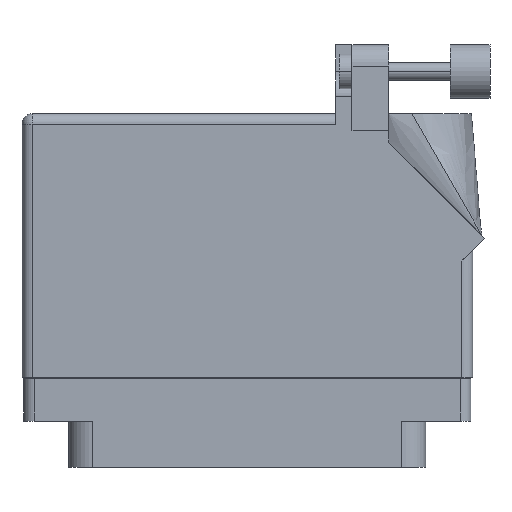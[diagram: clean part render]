
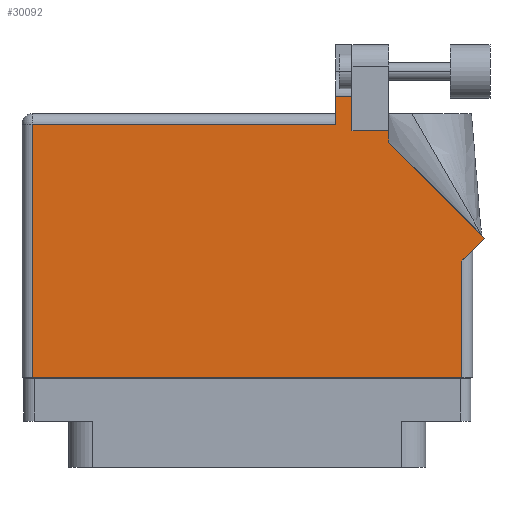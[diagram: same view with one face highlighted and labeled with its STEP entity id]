
A CAD part, front view. The second image highlights one B-rep face of the part: STEP entity #30092.
In plain terms, the highlighted face is planar.
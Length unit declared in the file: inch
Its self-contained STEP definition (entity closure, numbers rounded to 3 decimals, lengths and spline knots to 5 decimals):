
#143 = DIRECTION ( 'NONE',  ( -1., 0., 0. ) ) ;
#302 = EDGE_CURVE ( 'NONE', #26790, #39023, #39555, .T. ) ;
#1346 = EDGE_CURVE ( 'NONE', #25140, #21363, #42938, .T. ) ;
#1649 = EDGE_CURVE ( 'NONE', #23870, #14553, #26015, .T. ) ;
#1766 = ORIENTED_EDGE ( 'NONE', *, *, #33555, .T. ) ;
#2999 = ORIENTED_EDGE ( 'NONE', *, *, #47303, .T. ) ;
#3070 = DIRECTION ( 'NONE',  ( -1., 0., 0. ) ) ;
#3093 = EDGE_LOOP ( 'NONE', ( #38251, #18678, #31161, #1766, #7810, #27589, #23297, #26671, #46212, #2999, #3477 ) ) ;
#3477 = ORIENTED_EDGE ( 'NONE', *, *, #1346, .T. ) ;
#3501 = EDGE_CURVE ( 'NONE', #41612, #23870, #7761, .T. ) ;
#4159 = LINE ( 'NONE', #20643, #32594 ) ;
#5684 = LINE ( 'NONE', #46859, #42906 ) ;
#7761 = LINE ( 'NONE', #21615, #10096 ) ;
#7810 = ORIENTED_EDGE ( 'NONE', *, *, #3501, .T. ) ;
#8825 = CARTESIAN_POINT ( 'NONE',  ( 0.513, 1.5315, 0.455 ) ) ;
#8990 = CARTESIAN_POINT ( 'NONE',  ( 0.82, 1.33, 0.455 ) ) ;
#9104 = CARTESIAN_POINT ( 'NONE',  ( -1.306, -0.1, 0.455 ) ) ;
#10096 = VECTOR ( 'NONE', #36224, 39.37008 ) ;
#10325 = CARTESIAN_POINT ( 'NONE',  ( -1.306, 1.43, 0.455 ) ) ;
#10364 = LINE ( 'NONE', #22560, #47624 ) ;
#11052 = CARTESIAN_POINT ( 'NONE',  ( 0.513, 1.43, 0.455 ) ) ;
#11156 = CARTESIAN_POINT ( 'NONE',  ( 0.82, 1.33, 0.455 ) ) ;
#11971 = CARTESIAN_POINT ( 'NONE',  ( 0.607, 1.5315, 0.455 ) ) ;
#13573 = DIRECTION ( 'NONE',  ( 1., 0., 0. ) ) ;
#14553 = VERTEX_POINT ( 'NONE', #41869 ) ;
#15030 = DIRECTION ( 'NONE',  ( 0., -1., 0. ) ) ;
#15648 = VECTOR ( 'NONE', #45522, 39.37008 ) ;
#17263 = DIRECTION ( 'NONE',  ( -0.707, 0.707, 0. ) ) ;
#17900 = CARTESIAN_POINT ( 'NONE',  ( 1.37671, 0.70771, 0.455 ) ) ;
#18544 = DIRECTION ( 'NONE',  ( 0., 1., 0. ) ) ;
#18678 = ORIENTED_EDGE ( 'NONE', *, *, #45038, .T. ) ;
#19804 = VERTEX_POINT ( 'NONE', #17900 ) ;
#20394 = EDGE_CURVE ( 'NONE', #19804, #39127, #5684, .T. ) ;
#20643 = CARTESIAN_POINT ( 'NONE',  ( 0.93777, 1.5315, 0.455 ) ) ;
#20734 = CARTESIAN_POINT ( 'NONE',  ( 0.513, 1.368, 0.455 ) ) ;
#21363 = VERTEX_POINT ( 'NONE', #35754 ) ;
#21615 = CARTESIAN_POINT ( 'NONE',  ( -1.244, -0.1, 0.455 ) ) ;
#22560 = CARTESIAN_POINT ( 'NONE',  ( 0.607, 1.33, 0.455 ) ) ;
#23103 = VECTOR ( 'NONE', #13573, 39.37008 ) ;
#23297 = ORIENTED_EDGE ( 'NONE', *, *, #46153, .T. ) ;
#23406 = DIRECTION ( 'NONE',  ( -1., 0., 0. ) ) ;
#23870 = VERTEX_POINT ( 'NONE', #38397 ) ;
#24370 = VECTOR ( 'NONE', #15030, 39.37008 ) ;
#24628 = LINE ( 'NONE', #30578, #34501 ) ;
#25140 = VERTEX_POINT ( 'NONE', #8990 ) ;
#26015 = LINE ( 'NONE', #9104, #23103 ) ;
#26671 = ORIENTED_EDGE ( 'NONE', *, *, #31814, .T. ) ;
#26790 = VERTEX_POINT ( 'NONE', #8825 ) ;
#27062 = VECTOR ( 'NONE', #30600, 39.37008 ) ;
#27589 = ORIENTED_EDGE ( 'NONE', *, *, #1649, .T. ) ;
#27820 = CARTESIAN_POINT ( 'NONE',  ( 0.82, 1.26442, 0.455 ) ) ;
#27990 = DIRECTION ( 'NONE',  ( 0., 1., 0. ) ) ;
#29434 = VECTOR ( 'NONE', #27990, 39.37008 ) ;
#29480 = LINE ( 'NONE', #37997, #15648 ) ;
#30092 = ADVANCED_FACE ( 'NONE', ( #32371 ), #36321, .F. ) ;
#30578 = CARTESIAN_POINT ( 'NONE',  ( -1.306, 1.368, 0.455 ) ) ;
#30600 = DIRECTION ( 'NONE',  ( 0., 1., 0. ) ) ;
#31161 = ORIENTED_EDGE ( 'NONE', *, *, #302, .T. ) ;
#31619 = EDGE_CURVE ( 'NONE', #21363, #41381, #10364, .T. ) ;
#31814 = EDGE_CURVE ( 'NONE', #38472, #19804, #29480, .T. ) ;
#32371 = FACE_OUTER_BOUND ( 'NONE', #3093, .T. ) ;
#32594 = VECTOR ( 'NONE', #43076, 39.37008 ) ;
#32926 = LINE ( 'NONE', #34649, #27062 ) ;
#33509 = LINE ( 'NONE', #27820, #29434 ) ;
#33555 = EDGE_CURVE ( 'NONE', #39023, #41612, #24628, .T. ) ;
#34501 = VECTOR ( 'NONE', #23406, 39.37008 ) ;
#34649 = CARTESIAN_POINT ( 'NONE',  ( 1.244, 0.637, 0.455 ) ) ;
#35754 = CARTESIAN_POINT ( 'NONE',  ( 0.607, 1.33, 0.455 ) ) ;
#36224 = DIRECTION ( 'NONE',  ( 0., -1., 0. ) ) ;
#36321 = PLANE ( 'NONE',  #43887 ) ;
#37997 = CARTESIAN_POINT ( 'NONE',  ( 1.306, 0.637, 0.455 ) ) ;
#38251 = ORIENTED_EDGE ( 'NONE', *, *, #31619, .T. ) ;
#38397 = CARTESIAN_POINT ( 'NONE',  ( -1.244, -0.1, 0.455 ) ) ;
#38472 = VERTEX_POINT ( 'NONE', #39801 ) ;
#38820 = VECTOR ( 'NONE', #143, 39.37008 ) ;
#39023 = VERTEX_POINT ( 'NONE', #20734 ) ;
#39127 = VERTEX_POINT ( 'NONE', #44292 ) ;
#39555 = LINE ( 'NONE', #11052, #24370 ) ;
#39801 = CARTESIAN_POINT ( 'NONE',  ( 1.244, 0.575, 0.455 ) ) ;
#41381 = VERTEX_POINT ( 'NONE', #11971 ) ;
#41612 = VERTEX_POINT ( 'NONE', #47549 ) ;
#41869 = CARTESIAN_POINT ( 'NONE',  ( 1.244, -0.1, 0.455 ) ) ;
#42906 = VECTOR ( 'NONE', #17263, 39.37008 ) ;
#42938 = LINE ( 'NONE', #11156, #38820 ) ;
#43076 = DIRECTION ( 'NONE',  ( -1., 0., 0. ) ) ;
#43887 = AXIS2_PLACEMENT_3D ( 'NONE', #10325, #47592, #3070 ) ;
#44292 = CARTESIAN_POINT ( 'NONE',  ( 0.82, 1.26442, 0.455 ) ) ;
#45038 = EDGE_CURVE ( 'NONE', #41381, #26790, #4159, .T. ) ;
#45522 = DIRECTION ( 'NONE',  ( 0.707, 0.707, 0. ) ) ;
#46153 = EDGE_CURVE ( 'NONE', #14553, #38472, #32926, .T. ) ;
#46212 = ORIENTED_EDGE ( 'NONE', *, *, #20394, .T. ) ;
#46859 = CARTESIAN_POINT ( 'NONE',  ( 1.37671, 0.70771, 0.455 ) ) ;
#47303 = EDGE_CURVE ( 'NONE', #39127, #25140, #33509, .T. ) ;
#47549 = CARTESIAN_POINT ( 'NONE',  ( -1.244, 1.368, 0.455 ) ) ;
#47592 = DIRECTION ( 'NONE',  ( 0., 0., -1. ) ) ;
#47624 = VECTOR ( 'NONE', #18544, 39.37008 ) ;
